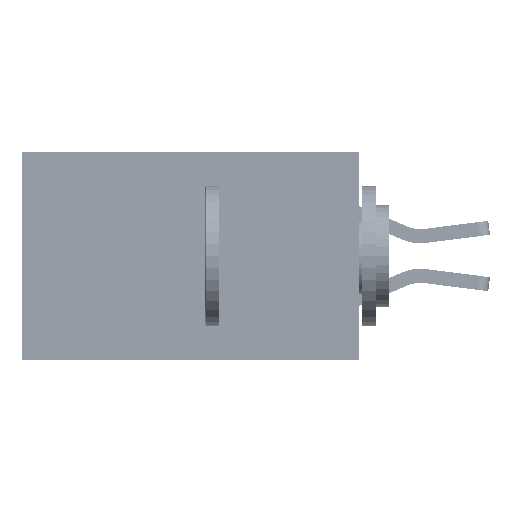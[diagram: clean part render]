
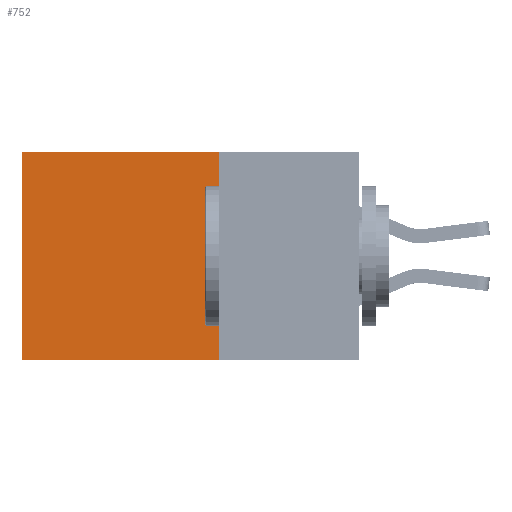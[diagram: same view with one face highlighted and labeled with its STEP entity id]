
A CAD part, left-side view. The second image highlights one B-rep face of the part: STEP entity #752.
In plain terms, the highlighted planar face has unit normal (-1, 0, 0).
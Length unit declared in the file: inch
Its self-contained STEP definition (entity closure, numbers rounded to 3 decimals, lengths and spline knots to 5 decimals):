
#752 = ADVANCED_FACE ( 'NONE', ( #11542 ), #32206, .F. ) ;
#1206 = EDGE_CURVE ( 'NONE', #22473, #16290, #21885, .T. ) ;
#3789 = VERTEX_POINT ( 'NONE', #29486 ) ;
#4243 = CARTESIAN_POINT ( 'NONE',  ( 0.2875, 0.25, 0. ) ) ;
#4707 = ORIENTED_EDGE ( 'NONE', *, *, #14304, .T. ) ;
#7504 = CARTESIAN_POINT ( 'NONE',  ( 0.2875, 0.25, -0.37 ) ) ;
#11542 = FACE_OUTER_BOUND ( 'NONE', #32226, .T. ) ;
#11630 = DIRECTION ( 'NONE',  ( 0., 1., 0. ) ) ;
#12652 = CARTESIAN_POINT ( 'NONE',  ( 0.2875, 0.6, 0. ) ) ;
#13000 = DIRECTION ( 'NONE',  ( 0., 0., -1. ) ) ;
#13297 = VECTOR ( 'NONE', #13000, 39.37008 ) ;
#14013 = CARTESIAN_POINT ( 'NONE',  ( 0.2875, 0.25, 0. ) ) ;
#14304 = EDGE_CURVE ( 'NONE', #40380, #3789, #29349, .T. ) ;
#15346 = DIRECTION ( 'NONE',  ( 0., 1., 0. ) ) ;
#16290 = VERTEX_POINT ( 'NONE', #7504 ) ;
#19764 = DIRECTION ( 'NONE',  ( 0., 0., -1. ) ) ;
#19831 = VECTOR ( 'NONE', #11630, 39.37008 ) ;
#19871 = LINE ( 'NONE', #4243, #33655 ) ;
#21879 = ORIENTED_EDGE ( 'NONE', *, *, #27594, .F. ) ;
#21885 = LINE ( 'NONE', #35043, #33345 ) ;
#22473 = VERTEX_POINT ( 'NONE', #14013 ) ;
#24384 = CARTESIAN_POINT ( 'NONE',  ( 0.2875, 0.6, 0. ) ) ;
#25003 = ORIENTED_EDGE ( 'NONE', *, *, #36968, .T. ) ;
#26749 = LINE ( 'NONE', #34278, #19831 ) ;
#27594 = EDGE_CURVE ( 'NONE', #16290, #3789, #26749, .T. ) ;
#28806 = DIRECTION ( 'NONE',  ( 0., 0., -1. ) ) ;
#29349 = LINE ( 'NONE', #24384, #13297 ) ;
#29486 = CARTESIAN_POINT ( 'NONE',  ( 0.2875, 0.6, -0.37 ) ) ;
#32206 = PLANE ( 'NONE',  #44083 ) ;
#32226 = EDGE_LOOP ( 'NONE', ( #4707, #21879, #36905, #25003 ) ) ;
#33345 = VECTOR ( 'NONE', #19764, 39.37008 ) ;
#33655 = VECTOR ( 'NONE', #15346, 39.37008 ) ;
#34278 = CARTESIAN_POINT ( 'NONE',  ( 0.2875, 0.25, -0.37 ) ) ;
#35043 = CARTESIAN_POINT ( 'NONE',  ( 0.2875, 0.25, 0. ) ) ;
#36066 = CARTESIAN_POINT ( 'NONE',  ( 0.2875, 0.25, 0. ) ) ;
#36905 = ORIENTED_EDGE ( 'NONE', *, *, #1206, .F. ) ;
#36968 = EDGE_CURVE ( 'NONE', #22473, #40380, #19871, .T. ) ;
#39629 = DIRECTION ( 'NONE',  ( 1., 0., 0. ) ) ;
#40380 = VERTEX_POINT ( 'NONE', #12652 ) ;
#44083 = AXIS2_PLACEMENT_3D ( 'NONE', #36066, #39629, #28806 ) ;
